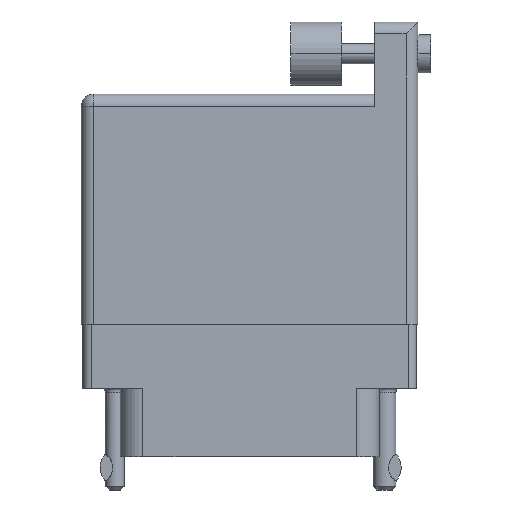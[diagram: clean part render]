
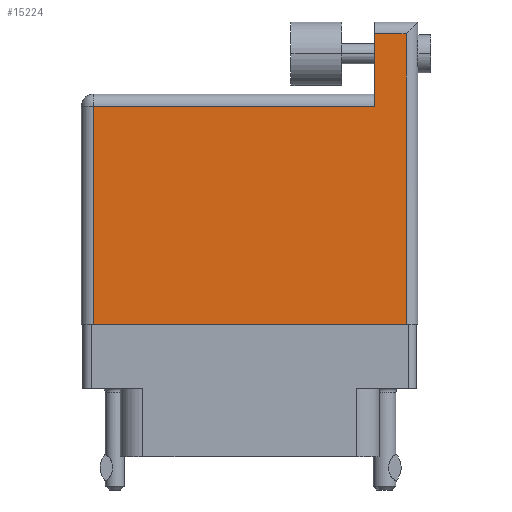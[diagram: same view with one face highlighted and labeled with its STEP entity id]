
A CAD part, front view. The second image highlights one B-rep face of the part: STEP entity #15224.
In plain terms, the highlighted face is planar.
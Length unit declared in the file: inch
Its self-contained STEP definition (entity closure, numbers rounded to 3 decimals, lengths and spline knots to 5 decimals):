
#267 = CARTESIAN_POINT ( 'NONE',  ( 0., 0.906, 0. ) ) ;
#431 = ORIENTED_EDGE ( 'NONE', *, *, #26301, .T. ) ;
#464 = EDGE_LOOP ( 'NONE', ( #2561, #25310, #30113, #30859, #431, #4807 ) ) ;
#674 = LINE ( 'NONE', #7509, #14078 ) ;
#2176 = DIRECTION ( 'NONE',  ( 0., -1., 0. ) ) ;
#2519 = FACE_OUTER_BOUND ( 'NONE', #464, .T. ) ;
#2561 = ORIENTED_EDGE ( 'NONE', *, *, #31738, .T. ) ;
#3021 = LINE ( 'NONE', #34557, #9093 ) ;
#3424 = DIRECTION ( 'NONE',  ( -1., 0., 0. ) ) ;
#4807 = ORIENTED_EDGE ( 'NONE', *, *, #13896, .T. ) ;
#5099 = CARTESIAN_POINT ( 'NONE',  ( 0.047, 0., 0. ) ) ;
#5290 = DIRECTION ( 'NONE',  ( 0., 1., 0. ) ) ;
#6081 = VERTEX_POINT ( 'NONE', #5099 ) ;
#6083 = EDGE_CURVE ( 'NONE', #35632, #23658, #674, .T. ) ;
#6309 = PLANE ( 'NONE',  #19185 ) ;
#6463 = VECTOR ( 'NONE', #20534, 39.37008 ) ;
#6659 = CARTESIAN_POINT ( 'NONE',  ( 0.047, 0., 0. ) ) ;
#6776 = VERTEX_POINT ( 'NONE', #26579 ) ;
#6904 = DIRECTION ( 'NONE',  ( -1., 0., 0. ) ) ;
#7104 = LINE ( 'NONE', #15792, #8860 ) ;
#7509 = CARTESIAN_POINT ( 'NONE',  ( 1.155, 1.19, 0. ) ) ;
#7907 = VERTEX_POINT ( 'NONE', #29653 ) ;
#8860 = VECTOR ( 'NONE', #5290, 39.37008 ) ;
#9093 = VECTOR ( 'NONE', #6904, 39.37008 ) ;
#9115 = DIRECTION ( 'NONE',  ( -1., 0., 0. ) ) ;
#10968 = VERTEX_POINT ( 'NONE', #15407 ) ;
#11633 = VECTOR ( 'NONE', #9115, 39.37008 ) ;
#13113 = VECTOR ( 'NONE', #20241, 39.37008 ) ;
#13340 = LINE ( 'NONE', #24913, #11633 ) ;
#13896 = EDGE_CURVE ( 'NONE', #10968, #6081, #18968, .T. ) ;
#14078 = VECTOR ( 'NONE', #2176, 39.37008 ) ;
#15224 = ADVANCED_FACE ( 'NONE', ( #2519 ), #6309, .F. ) ;
#15407 = CARTESIAN_POINT ( 'NONE',  ( 0.047, 0.859, 0. ) ) ;
#15792 = CARTESIAN_POINT ( 'NONE',  ( 1.278, 1.19, 0. ) ) ;
#18968 = LINE ( 'NONE', #6659, #6463 ) ;
#19185 = AXIS2_PLACEMENT_3D ( 'NONE', #267, #19959, #3424 ) ;
#19898 = CARTESIAN_POINT ( 'NONE',  ( 0., 0., 0. ) ) ;
#19959 = DIRECTION ( 'NONE',  ( 0., 0., -1. ) ) ;
#20241 = DIRECTION ( 'NONE',  ( 1., 0., 0. ) ) ;
#20534 = DIRECTION ( 'NONE',  ( 0., -1., 0. ) ) ;
#22869 = EDGE_CURVE ( 'NONE', #7907, #35632, #3021, .T. ) ;
#23658 = VERTEX_POINT ( 'NONE', #31685 ) ;
#24913 = CARTESIAN_POINT ( 'NONE',  ( 0., 0.859, 0. ) ) ;
#25310 = ORIENTED_EDGE ( 'NONE', *, *, #33471, .T. ) ;
#26301 = EDGE_CURVE ( 'NONE', #23658, #10968, #13340, .T. ) ;
#26579 = CARTESIAN_POINT ( 'NONE',  ( 1.278, 0., 0. ) ) ;
#29653 = CARTESIAN_POINT ( 'NONE',  ( 1.278, 1.143, 0. ) ) ;
#30113 = ORIENTED_EDGE ( 'NONE', *, *, #22869, .T. ) ;
#30859 = ORIENTED_EDGE ( 'NONE', *, *, #6083, .T. ) ;
#31685 = CARTESIAN_POINT ( 'NONE',  ( 1.155, 0.859, 0. ) ) ;
#31738 = EDGE_CURVE ( 'NONE', #6081, #6776, #33884, .T. ) ;
#33471 = EDGE_CURVE ( 'NONE', #6776, #7907, #7104, .T. ) ;
#33884 = LINE ( 'NONE', #19898, #13113 ) ;
#34557 = CARTESIAN_POINT ( 'NONE',  ( 1.155, 1.143, 0. ) ) ;
#34745 = CARTESIAN_POINT ( 'NONE',  ( 1.155, 1.143, 0. ) ) ;
#35632 = VERTEX_POINT ( 'NONE', #34745 ) ;
